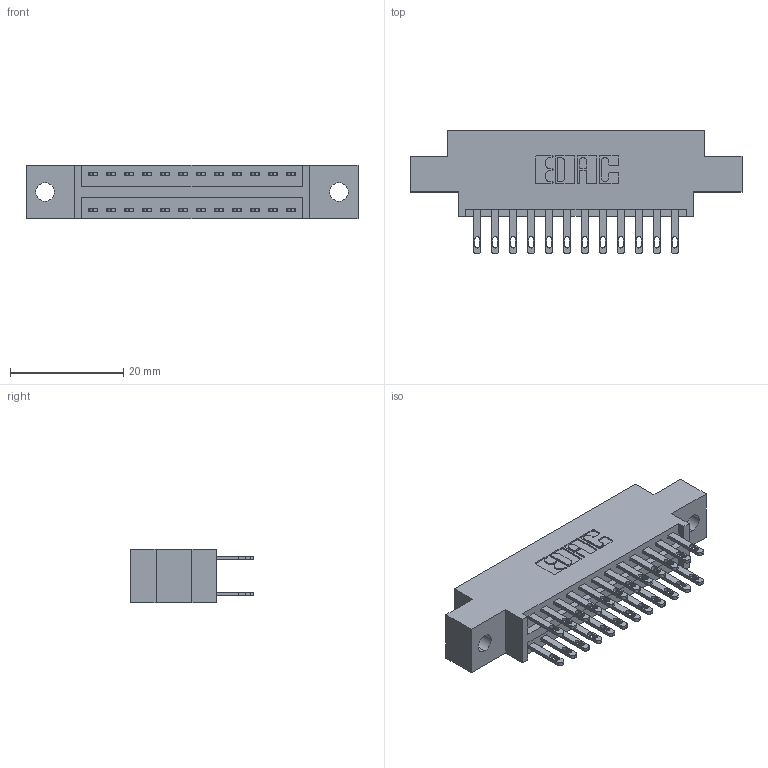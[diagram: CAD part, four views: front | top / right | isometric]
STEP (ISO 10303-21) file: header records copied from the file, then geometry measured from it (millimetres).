
FILE_DESCRIPTION (( 'STEP AP203' ), '1' );
FILE_NAME ('896-024-500-802.STEP', '2021-07-27T17:32:56', ( '' ), ( '' ), 'SwSTEP 2.0', 'SolidWorks 2020', '' );
FILE_SCHEMA (( 'CONFIG_CONTROL_DESIGN' ));
Length unit declared in the file: inch
Products named in the file (3): 846 Part_0.170 Offset - 0.128 Dia; 345-292-001_345-293-100; 896-024-500-802
Assembly tree (25 placements, depth 2):
  896-024-500-802
    846 Part_0.170 Offset - 0.128 Dia
    345-292-001_345-293-100  x24
Bounding box: 58.67 x 21.84 x 9.4 mm (x, y, z)
Volume: 5370.5 mm3; surface area: 7072.1 mm2
Topology: 25 solids, 25 shells, 1278 faces, 3869 edges, 2578 vertices
Faces by surface type: plane 776, cylinder 502
Entity records: 11935 total; most frequent: CARTESIAN_POINT 2008, ORIENTED_EDGE 1942, DIRECTION 1823, EDGE_CURVE 971, LINE 787, VECTOR 787, VERTEX_POINT 646, AXIS2_PLACEMENT_3D 518
